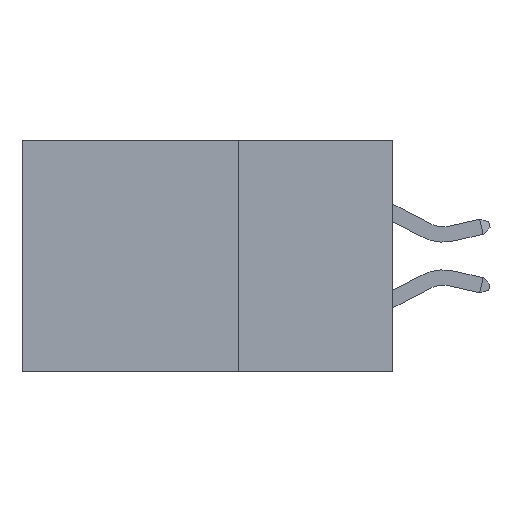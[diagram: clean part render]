
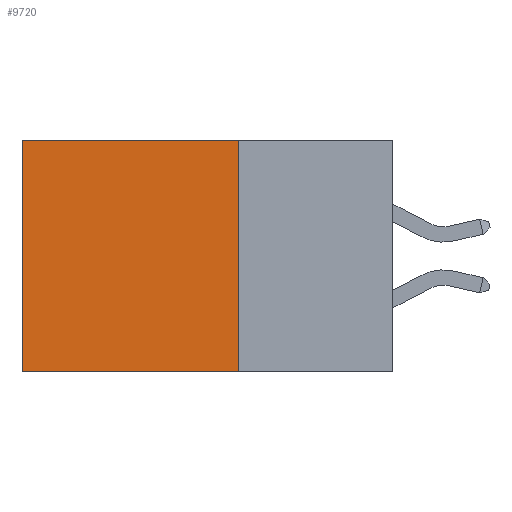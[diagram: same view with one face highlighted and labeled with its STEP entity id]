
A CAD part, left-side view. The second image highlights one B-rep face of the part: STEP entity #9720.
In plain terms, the highlighted planar face has unit normal (-1, 0, 0).
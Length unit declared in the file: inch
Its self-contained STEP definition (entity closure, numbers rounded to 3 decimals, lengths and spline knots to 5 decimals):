
#115 = LINE ( 'NONE', #8056, #586 ) ;
#116 = CARTESIAN_POINT ( 'NONE',  ( 0.2875, 0.25, 0. ) ) ;
#144 = AXIS2_PLACEMENT_3D ( 'NONE', #8837, #4983, #2577 ) ;
#450 = EDGE_LOOP ( 'NONE', ( #9126, #9494, #4371, #3022 ) ) ;
#586 = VECTOR ( 'NONE', #1826, 39.37008 ) ;
#739 = LINE ( 'NONE', #8520, #9255 ) ;
#864 = CARTESIAN_POINT ( 'NONE',  ( 0.2875, 0.25, 0. ) ) ;
#1826 = DIRECTION ( 'NONE',  ( 0., 0., -1. ) ) ;
#2332 = VECTOR ( 'NONE', #7804, 39.37008 ) ;
#2577 = DIRECTION ( 'NONE',  ( 0., 0., -1. ) ) ;
#3022 = ORIENTED_EDGE ( 'NONE', *, *, #7964, .T. ) ;
#3070 = CARTESIAN_POINT ( 'NONE',  ( 0.2875, 0.6, 0. ) ) ;
#3235 = FACE_OUTER_BOUND ( 'NONE', #450, .T. ) ;
#3539 = VERTEX_POINT ( 'NONE', #7975 ) ;
#3611 = CARTESIAN_POINT ( 'NONE',  ( 0.2875, 0.6, -0.375 ) ) ;
#4102 = LINE ( 'NONE', #5568, #2332 ) ;
#4371 = ORIENTED_EDGE ( 'NONE', *, *, #7917, .F. ) ;
#4692 = DIRECTION ( 'NONE',  ( 0., 0., -1. ) ) ;
#4983 = DIRECTION ( 'NONE',  ( 1., 0., 0. ) ) ;
#5568 = CARTESIAN_POINT ( 'NONE',  ( 0.2875, 0.25, -0.375 ) ) ;
#6019 = VERTEX_POINT ( 'NONE', #3070 ) ;
#6126 = VECTOR ( 'NONE', #6945, 39.37008 ) ;
#6794 = EDGE_CURVE ( 'NONE', #3539, #8716, #4102, .T. ) ;
#6945 = DIRECTION ( 'NONE',  ( 0., 1., 0. ) ) ;
#7804 = DIRECTION ( 'NONE',  ( 0., 1., 0. ) ) ;
#7917 = EDGE_CURVE ( 'NONE', #8220, #3539, #739, .T. ) ;
#7925 = LINE ( 'NONE', #116, #6126 ) ;
#7964 = EDGE_CURVE ( 'NONE', #8220, #6019, #7925, .T. ) ;
#7975 = CARTESIAN_POINT ( 'NONE',  ( 0.2875, 0.25, -0.375 ) ) ;
#8056 = CARTESIAN_POINT ( 'NONE',  ( 0.2875, 0.6, -0.375 ) ) ;
#8220 = VERTEX_POINT ( 'NONE', #864 ) ;
#8520 = CARTESIAN_POINT ( 'NONE',  ( 0.2875, 0.25, -0.375 ) ) ;
#8716 = VERTEX_POINT ( 'NONE', #3611 ) ;
#8837 = CARTESIAN_POINT ( 'NONE',  ( 0.2875, 0.25, -0.375 ) ) ;
#9126 = ORIENTED_EDGE ( 'NONE', *, *, #9795, .T. ) ;
#9255 = VECTOR ( 'NONE', #4692, 39.37008 ) ;
#9488 = PLANE ( 'NONE',  #144 ) ;
#9494 = ORIENTED_EDGE ( 'NONE', *, *, #6794, .F. ) ;
#9720 = ADVANCED_FACE ( 'NONE', ( #3235 ), #9488, .F. ) ;
#9795 = EDGE_CURVE ( 'NONE', #6019, #8716, #115, .T. ) ;
